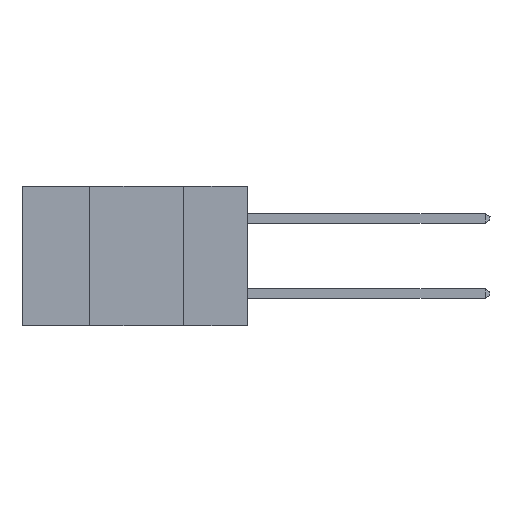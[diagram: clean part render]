
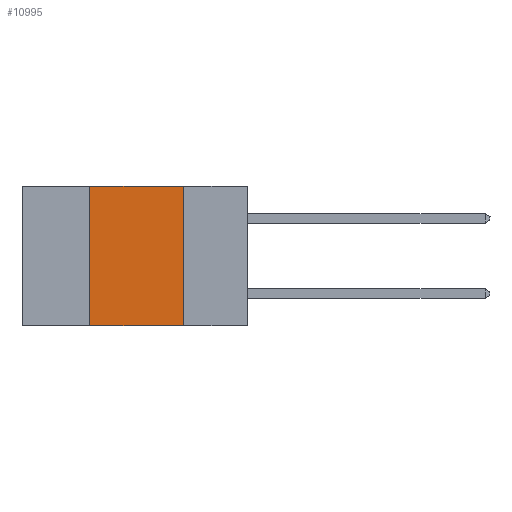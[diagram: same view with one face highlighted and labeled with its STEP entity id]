
A CAD part, left-side view. The second image highlights one B-rep face of the part: STEP entity #10995.
In plain terms, the highlighted planar face has unit normal (-1, 0, 0).
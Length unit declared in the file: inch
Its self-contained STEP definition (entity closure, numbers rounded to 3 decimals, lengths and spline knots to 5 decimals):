
#480 = CARTESIAN_POINT ( 'NONE',  ( 0., 0.6, -0.37 ) ) ;
#986 = DIRECTION ( 'NONE',  ( 0., 0., 1. ) ) ;
#1060 = ORIENTED_EDGE ( 'NONE', *, *, #3345, .F. ) ;
#1930 = CARTESIAN_POINT ( 'NONE',  ( 0., 0.17, -0.37 ) ) ;
#1988 = VECTOR ( 'NONE', #17697, 39.37008 ) ;
#2212 = LINE ( 'NONE', #5685, #1988 ) ;
#2727 = ORIENTED_EDGE ( 'NONE', *, *, #3125, .F. ) ;
#3066 = EDGE_CURVE ( 'NONE', #16266, #17204, #8023, .T. ) ;
#3125 = EDGE_CURVE ( 'NONE', #16266, #4674, #15416, .T. ) ;
#3345 = EDGE_CURVE ( 'NONE', #4674, #6095, #13315, .T. ) ;
#3977 = ORIENTED_EDGE ( 'NONE', *, *, #13065, .F. ) ;
#4674 = VERTEX_POINT ( 'NONE', #11258 ) ;
#5597 = CARTESIAN_POINT ( 'NONE',  ( 0., 0.42, 0. ) ) ;
#5685 = CARTESIAN_POINT ( 'NONE',  ( 0., 0.17, 0. ) ) ;
#6095 = VERTEX_POINT ( 'NONE', #14378 ) ;
#7106 = AXIS2_PLACEMENT_3D ( 'NONE', #15122, #12280, #11048 ) ;
#7654 = CARTESIAN_POINT ( 'NONE',  ( 0., 0.6, 0. ) ) ;
#7998 = DIRECTION ( 'NONE',  ( 0., -1., 0. ) ) ;
#8023 = LINE ( 'NONE', #480, #12413 ) ;
#8106 = DIRECTION ( 'NONE',  ( 0., -1., 0. ) ) ;
#8630 = EDGE_LOOP ( 'NONE', ( #3977, #1060, #2727, #11738 ) ) ;
#10995 = ADVANCED_FACE ( 'NONE', ( #18580 ), #16370, .F. ) ;
#11048 = DIRECTION ( 'NONE',  ( 0., 0., -1. ) ) ;
#11258 = CARTESIAN_POINT ( 'NONE',  ( 0., 0.42, 0. ) ) ;
#11738 = ORIENTED_EDGE ( 'NONE', *, *, #3066, .T. ) ;
#12109 = CARTESIAN_POINT ( 'NONE',  ( 0., 0.42, -0.37 ) ) ;
#12280 = DIRECTION ( 'NONE',  ( 1., 0., 0. ) ) ;
#12413 = VECTOR ( 'NONE', #7998, 39.37008 ) ;
#13065 = EDGE_CURVE ( 'NONE', #6095, #17204, #2212, .T. ) ;
#13315 = LINE ( 'NONE', #7654, #17044 ) ;
#14378 = CARTESIAN_POINT ( 'NONE',  ( 0., 0.17, 0. ) ) ;
#15122 = CARTESIAN_POINT ( 'NONE',  ( 0., 0.6, 0. ) ) ;
#15416 = LINE ( 'NONE', #5597, #18861 ) ;
#16266 = VERTEX_POINT ( 'NONE', #12109 ) ;
#16370 = PLANE ( 'NONE',  #7106 ) ;
#17044 = VECTOR ( 'NONE', #8106, 39.37008 ) ;
#17204 = VERTEX_POINT ( 'NONE', #1930 ) ;
#17697 = DIRECTION ( 'NONE',  ( 0., 0., -1. ) ) ;
#18580 = FACE_OUTER_BOUND ( 'NONE', #8630, .T. ) ;
#18861 = VECTOR ( 'NONE', #986, 39.37008 ) ;
